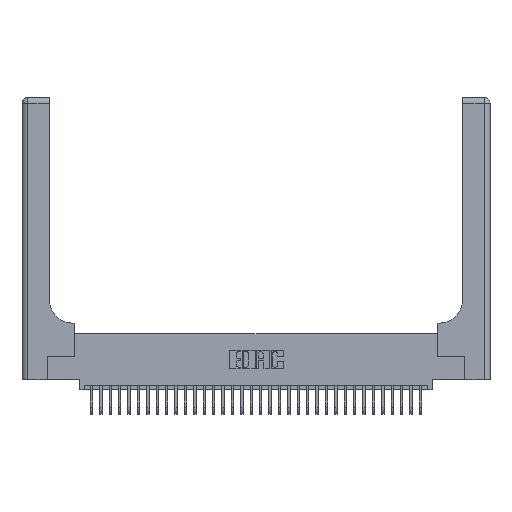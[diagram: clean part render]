
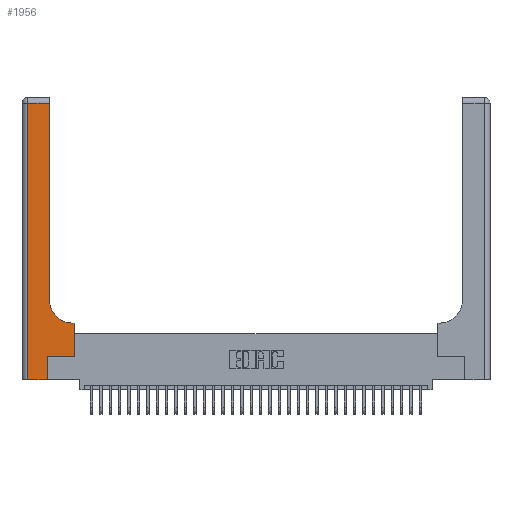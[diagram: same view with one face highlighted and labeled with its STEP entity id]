
A CAD part, top view. The second image highlights one B-rep face of the part: STEP entity #1956.
In plain terms, the highlighted planar face has unit normal (0, 0, 1).
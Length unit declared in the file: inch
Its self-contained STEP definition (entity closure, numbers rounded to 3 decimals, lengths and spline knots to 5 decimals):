
#76 = ORIENTED_EDGE ( 'NONE', *, *, #13258, .T. ) ;
#229 = CARTESIAN_POINT ( 'NONE',  ( 0.2915, 0.85, 0.37 ) ) ;
#230 = DIRECTION ( 'NONE',  ( 1., 0., 0. ) ) ;
#610 = AXIS2_PLACEMENT_3D ( 'NONE', #31024, #15741, #230 ) ;
#1108 = VERTEX_POINT ( 'NONE', #5291 ) ;
#1274 = VECTOR ( 'NONE', #13976, 39.37008 ) ;
#1956 = ADVANCED_FACE ( 'NONE', ( #3476 ), #27341, .F. ) ;
#2335 = EDGE_LOOP ( 'NONE', ( #76, #2870, #28217, #32459, #18998, #22824, #13412, #31870, #6157 ) ) ;
#2421 = CARTESIAN_POINT ( 'NONE',  ( 0.5585, 0.25, 0.37 ) ) ;
#2870 = ORIENTED_EDGE ( 'NONE', *, *, #6883, .T. ) ;
#3142 = EDGE_CURVE ( 'NONE', #10620, #13837, #23925, .T. ) ;
#3165 = LINE ( 'NONE', #30992, #29684 ) ;
#3476 = FACE_OUTER_BOUND ( 'NONE', #2335, .T. ) ;
#4188 = EDGE_CURVE ( 'NONE', #30475, #28075, #26297, .T. ) ;
#5261 = DIRECTION ( 'NONE',  ( 1., 0., 0. ) ) ;
#5291 = CARTESIAN_POINT ( 'NONE',  ( 0.269, 0., 0.37 ) ) ;
#6157 = ORIENTED_EDGE ( 'NONE', *, *, #10775, .T. ) ;
#6883 = EDGE_CURVE ( 'NONE', #23982, #10620, #21725, .T. ) ;
#6965 = CARTESIAN_POINT ( 'NONE',  ( 0.2915, 0.6, 0.37 ) ) ;
#7235 = VECTOR ( 'NONE', #10436, 39.37008 ) ;
#7451 = EDGE_CURVE ( 'NONE', #1108, #16744, #3165, .T. ) ;
#7619 = DIRECTION ( 'NONE',  ( 0., 1., 0. ) ) ;
#7998 = DIRECTION ( 'NONE',  ( 0., 1., 0. ) ) ;
#9806 = LINE ( 'NONE', #11359, #1274 ) ;
#10436 = DIRECTION ( 'NONE',  ( -1., 0., 0. ) ) ;
#10620 = VERTEX_POINT ( 'NONE', #12255 ) ;
#10775 = EDGE_CURVE ( 'NONE', #28075, #20560, #10912, .T. ) ;
#10912 = CIRCLE ( 'NONE', #610, 0.25 ) ;
#11359 = CARTESIAN_POINT ( 'NONE',  ( 0.269, 0.25, 0.37 ) ) ;
#11580 = CARTESIAN_POINT ( 'NONE',  ( 0.06, 0., 0.37 ) ) ;
#11614 = CARTESIAN_POINT ( 'NONE',  ( 0.06, 3., 0.37 ) ) ;
#12255 = CARTESIAN_POINT ( 'NONE',  ( 0.06, 2.94, 0.37 ) ) ;
#12439 = CARTESIAN_POINT ( 'NONE',  ( 0.5585, 0.25, 0.37 ) ) ;
#12892 = VECTOR ( 'NONE', #7619, 39.37008 ) ;
#13258 = EDGE_CURVE ( 'NONE', #20560, #23982, #17613, .T. ) ;
#13412 = ORIENTED_EDGE ( 'NONE', *, *, #29677, .T. ) ;
#13524 = VECTOR ( 'NONE', #24918, 39.37008 ) ;
#13837 = VERTEX_POINT ( 'NONE', #11580 ) ;
#13976 = DIRECTION ( 'NONE',  ( 1., 0., 0. ) ) ;
#14622 = DIRECTION ( 'NONE',  ( -1., 0., 0. ) ) ;
#15741 = DIRECTION ( 'NONE',  ( 0., 0., -1. ) ) ;
#16396 = EDGE_CURVE ( 'NONE', #16744, #25039, #9806, .T. ) ;
#16744 = VERTEX_POINT ( 'NONE', #33294 ) ;
#16784 = DIRECTION ( 'NONE',  ( 0., 1., 0. ) ) ;
#17613 = LINE ( 'NONE', #26942, #30417 ) ;
#18488 = CARTESIAN_POINT ( 'NONE',  ( 0.5585, 0.6, 0.37 ) ) ;
#18998 = ORIENTED_EDGE ( 'NONE', *, *, #7451, .T. ) ;
#19540 = VECTOR ( 'NONE', #5261, 39.37008 ) ;
#20231 = CARTESIAN_POINT ( 'NONE',  ( 0.2915, 2.94, 0.37 ) ) ;
#20560 = VERTEX_POINT ( 'NONE', #229 ) ;
#21725 = LINE ( 'NONE', #28354, #7235 ) ;
#22497 = AXIS2_PLACEMENT_3D ( 'NONE', #24777, #29938, #14622 ) ;
#22824 = ORIENTED_EDGE ( 'NONE', *, *, #16396, .T. ) ;
#23252 = CARTESIAN_POINT ( 'NONE',  ( 0., 0., 0.37 ) ) ;
#23925 = LINE ( 'NONE', #11614, #29941 ) ;
#23982 = VERTEX_POINT ( 'NONE', #20231 ) ;
#24370 = DIRECTION ( 'NONE',  ( 0., -1., 0. ) ) ;
#24777 = CARTESIAN_POINT ( 'NONE',  ( 0., 3., 0.37 ) ) ;
#24918 = DIRECTION ( 'NONE',  ( -1., 0., 0. ) ) ;
#25039 = VERTEX_POINT ( 'NONE', #12439 ) ;
#26297 = LINE ( 'NONE', #6965, #13524 ) ;
#26942 = CARTESIAN_POINT ( 'NONE',  ( 0.2915, 3., 0.37 ) ) ;
#27110 = CARTESIAN_POINT ( 'NONE',  ( 0.5415, 0.6, 0.37 ) ) ;
#27341 = PLANE ( 'NONE',  #22497 ) ;
#28075 = VERTEX_POINT ( 'NONE', #27110 ) ;
#28217 = ORIENTED_EDGE ( 'NONE', *, *, #3142, .T. ) ;
#28354 = CARTESIAN_POINT ( 'NONE',  ( 0., 2.94, 0.37 ) ) ;
#28733 = LINE ( 'NONE', #23252, #19540 ) ;
#29677 = EDGE_CURVE ( 'NONE', #25039, #30475, #33281, .T. ) ;
#29684 = VECTOR ( 'NONE', #7998, 39.37008 ) ;
#29938 = DIRECTION ( 'NONE',  ( 0., 0., -1. ) ) ;
#29941 = VECTOR ( 'NONE', #24370, 39.37008 ) ;
#30417 = VECTOR ( 'NONE', #16784, 39.37008 ) ;
#30475 = VERTEX_POINT ( 'NONE', #18488 ) ;
#30992 = CARTESIAN_POINT ( 'NONE',  ( 0.269, 0., 0.37 ) ) ;
#31024 = CARTESIAN_POINT ( 'NONE',  ( 0.5415, 0.85, 0.37 ) ) ;
#31858 = EDGE_CURVE ( 'NONE', #13837, #1108, #28733, .T. ) ;
#31870 = ORIENTED_EDGE ( 'NONE', *, *, #4188, .T. ) ;
#32459 = ORIENTED_EDGE ( 'NONE', *, *, #31858, .T. ) ;
#33281 = LINE ( 'NONE', #2421, #12892 ) ;
#33294 = CARTESIAN_POINT ( 'NONE',  ( 0.269, 0.25, 0.37 ) ) ;
